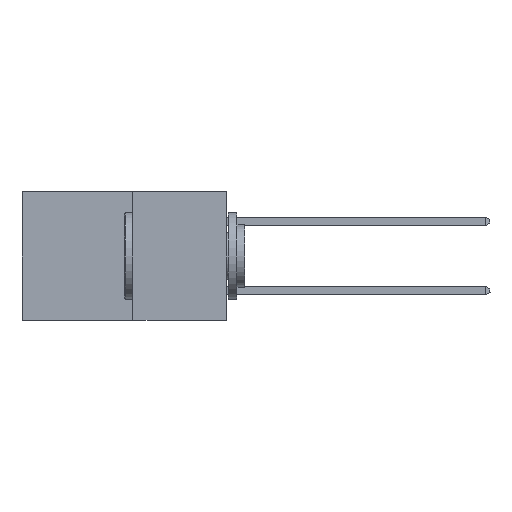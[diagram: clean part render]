
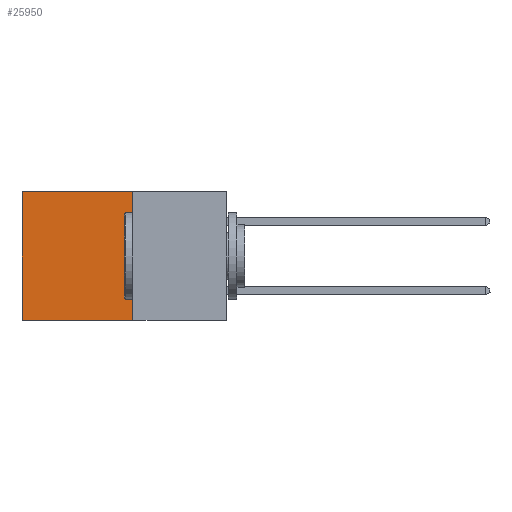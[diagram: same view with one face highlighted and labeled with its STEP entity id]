
A CAD part, left-side view. The second image highlights one B-rep face of the part: STEP entity #25950.
In plain terms, the highlighted planar face has unit normal (-1, 0, 0).
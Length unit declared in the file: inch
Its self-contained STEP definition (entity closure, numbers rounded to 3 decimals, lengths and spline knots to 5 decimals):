
#656 = LINE ( 'NONE', #15208, #1347 ) ;
#788 = LINE ( 'NONE', #25020, #12620 ) ;
#1347 = VECTOR ( 'NONE', #17433, 39.37008 ) ;
#1538 = DIRECTION ( 'NONE',  ( 0., 1., 0. ) ) ;
#2855 = DIRECTION ( 'NONE',  ( 0., 0., -1. ) ) ;
#5978 = ORIENTED_EDGE ( 'NONE', *, *, #12985, .F. ) ;
#6116 = LINE ( 'NONE', #24891, #11326 ) ;
#6971 = ORIENTED_EDGE ( 'NONE', *, *, #19930, .F. ) ;
#8120 = CARTESIAN_POINT ( 'NONE',  ( 0.277, 0.27, -0.37 ) ) ;
#8140 = CARTESIAN_POINT ( 'NONE',  ( 0.277, 0.27, 0. ) ) ;
#10376 = DIRECTION ( 'NONE',  ( 0., 0., -1. ) ) ;
#10709 = EDGE_CURVE ( 'NONE', #15234, #23420, #788, .T. ) ;
#10868 = EDGE_LOOP ( 'NONE', ( #19068, #6971, #5978, #11548 ) ) ;
#11326 = VECTOR ( 'NONE', #13874, 39.37008 ) ;
#11548 = ORIENTED_EDGE ( 'NONE', *, *, #18143, .T. ) ;
#12620 = VECTOR ( 'NONE', #2855, 39.37008 ) ;
#12985 = EDGE_CURVE ( 'NONE', #26954, #26745, #656, .T. ) ;
#13874 = DIRECTION ( 'NONE',  ( 0., 1., 0. ) ) ;
#15208 = CARTESIAN_POINT ( 'NONE',  ( 0.277, 0.27, -0.37 ) ) ;
#15234 = VERTEX_POINT ( 'NONE', #22007 ) ;
#15841 = CARTESIAN_POINT ( 'NONE',  ( 0.277, 0.27, 0. ) ) ;
#16963 = PLANE ( 'NONE',  #23600 ) ;
#17433 = DIRECTION ( 'NONE',  ( 0., 0., -1. ) ) ;
#18143 = EDGE_CURVE ( 'NONE', #26954, #15234, #27679, .T. ) ;
#19068 = ORIENTED_EDGE ( 'NONE', *, *, #10709, .T. ) ;
#19571 = FACE_OUTER_BOUND ( 'NONE', #10868, .T. ) ;
#19930 = EDGE_CURVE ( 'NONE', #26745, #23420, #6116, .T. ) ;
#21841 = VECTOR ( 'NONE', #1538, 39.37008 ) ;
#22007 = CARTESIAN_POINT ( 'NONE',  ( 0.277, 0.59, 0. ) ) ;
#23036 = CARTESIAN_POINT ( 'NONE',  ( 0.277, 0.59, -0.37 ) ) ;
#23420 = VERTEX_POINT ( 'NONE', #23036 ) ;
#23600 = AXIS2_PLACEMENT_3D ( 'NONE', #8120, #23631, #10376 ) ;
#23631 = DIRECTION ( 'NONE',  ( 1., 0., 0. ) ) ;
#24891 = CARTESIAN_POINT ( 'NONE',  ( 0.277, 0.27, -0.37 ) ) ;
#25020 = CARTESIAN_POINT ( 'NONE',  ( 0.277, 0.59, -0.37 ) ) ;
#25950 = ADVANCED_FACE ( 'NONE', ( #19571 ), #16963, .F. ) ;
#26745 = VERTEX_POINT ( 'NONE', #28347 ) ;
#26954 = VERTEX_POINT ( 'NONE', #15841 ) ;
#27679 = LINE ( 'NONE', #8140, #21841 ) ;
#28347 = CARTESIAN_POINT ( 'NONE',  ( 0.277, 0.27, -0.37 ) ) ;
